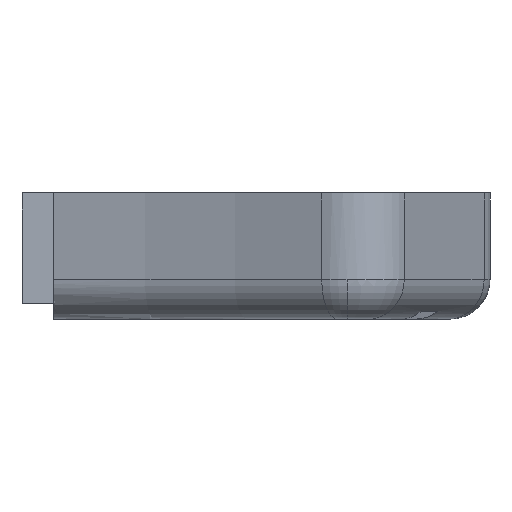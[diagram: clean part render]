
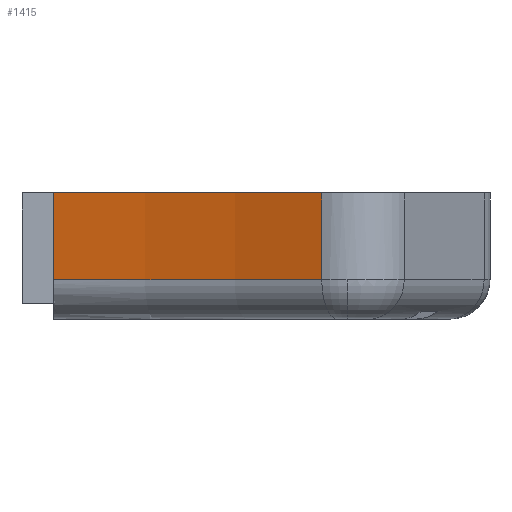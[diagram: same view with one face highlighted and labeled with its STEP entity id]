
A CAD part, left-side view. The second image highlights one B-rep face of the part: STEP entity #1415.
In plain terms, the highlighted cylindrical face has radius 155 mm (diameter 310 mm), a partial arc.
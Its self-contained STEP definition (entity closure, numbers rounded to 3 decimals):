
#27 = DIRECTION ( 'NONE',  ( 0., 0., 1. ) ) ;
#112 = AXIS2_PLACEMENT_3D ( 'NONE', #325, #1513, #490 ) ;
#117 = DIRECTION ( 'NONE',  ( 1., 0., 0. ) ) ;
#263 = FACE_OUTER_BOUND ( 'NONE', #783, .T. ) ;
#278 = EDGE_CURVE ( 'NONE', #548, #1636, #401, .T. ) ;
#314 = EDGE_CURVE ( 'NONE', #548, #2092, #1650, .T. ) ;
#325 = CARTESIAN_POINT ( 'NONE',  ( -175., 0., 0. ) ) ;
#355 = CARTESIAN_POINT ( 'NONE',  ( -175., 0., -17.6 ) ) ;
#390 = CARTESIAN_POINT ( 'NONE',  ( -22.55, -28., -11. ) ) ;
#400 = CARTESIAN_POINT ( 'NONE',  ( -22.55, -28., 0. ) ) ;
#401 = CIRCLE ( 'NONE', #593, 155. ) ;
#453 = EDGE_CURVE ( 'NONE', #733, #2092, #1780, .T. ) ;
#490 = DIRECTION ( 'NONE',  ( 1., 0., 0. ) ) ;
#548 = VERTEX_POINT ( 'NONE', #390 ) ;
#593 = AXIS2_PLACEMENT_3D ( 'NONE', #2123, #1115, #117 ) ;
#644 = DIRECTION ( 'NONE',  ( 0., 0., 1. ) ) ;
#733 = VERTEX_POINT ( 'NONE', #2138 ) ;
#783 = EDGE_LOOP ( 'NONE', ( #971, #978, #1080, #1405 ) ) ;
#897 = VECTOR ( 'NONE', #1641, 1000. ) ;
#901 = AXIS2_PLACEMENT_3D ( 'NONE', #355, #27, #1704 ) ;
#957 = CARTESIAN_POINT ( 'NONE',  ( -22.55, -28., -17.6 ) ) ;
#971 = ORIENTED_EDGE ( 'NONE', *, *, #314, .F. ) ;
#978 = ORIENTED_EDGE ( 'NONE', *, *, #278, .T. ) ;
#1080 = ORIENTED_EDGE ( 'NONE', *, *, #1526, .T. ) ;
#1100 = CYLINDRICAL_SURFACE ( 'NONE', #901, 155. ) ;
#1115 = DIRECTION ( 'NONE',  ( 0., 0., -1. ) ) ;
#1200 = VECTOR ( 'NONE', #644, 1000. ) ;
#1334 = CARTESIAN_POINT ( 'NONE',  ( -32.957, -62.039, -17.6 ) ) ;
#1351 = CARTESIAN_POINT ( 'NONE',  ( -32.957, -62.039, -11. ) ) ;
#1405 = ORIENTED_EDGE ( 'NONE', *, *, #453, .T. ) ;
#1415 = ADVANCED_FACE ( 'NONE', ( #263 ), #1100, .F. ) ;
#1513 = DIRECTION ( 'NONE',  ( 0., 0., 1. ) ) ;
#1526 = EDGE_CURVE ( 'NONE', #1636, #733, #1660, .T. ) ;
#1636 = VERTEX_POINT ( 'NONE', #1351 ) ;
#1641 = DIRECTION ( 'NONE',  ( 0., 0., 1. ) ) ;
#1650 = LINE ( 'NONE', #957, #897 ) ;
#1660 = LINE ( 'NONE', #1334, #1200 ) ;
#1704 = DIRECTION ( 'NONE',  ( 1., 0., 0. ) ) ;
#1780 = CIRCLE ( 'NONE', #112, 155. ) ;
#2092 = VERTEX_POINT ( 'NONE', #400 ) ;
#2123 = CARTESIAN_POINT ( 'NONE',  ( -175., 0., -11. ) ) ;
#2138 = CARTESIAN_POINT ( 'NONE',  ( -32.957, -62.039, 0. ) ) ;
